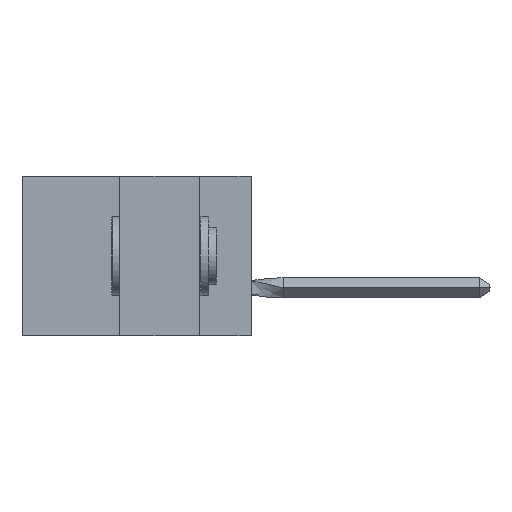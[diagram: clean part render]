
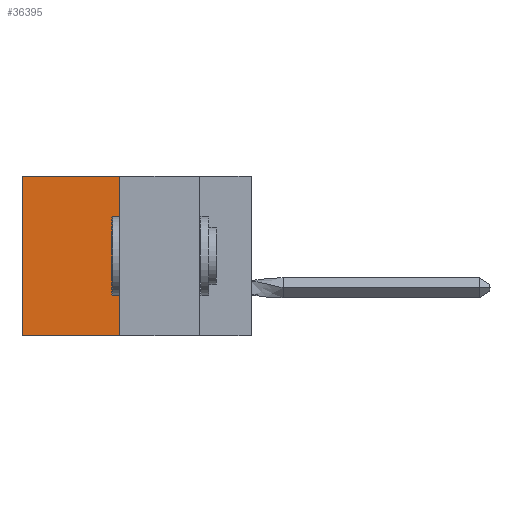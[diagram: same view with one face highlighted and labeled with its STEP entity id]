
A CAD part, left-side view. The second image highlights one B-rep face of the part: STEP entity #36395.
In plain terms, the highlighted planar face has unit normal (-1, 0, 0).
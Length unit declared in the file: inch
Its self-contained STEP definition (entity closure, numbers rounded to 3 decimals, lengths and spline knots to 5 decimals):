
#522 = ORIENTED_EDGE ( 'NONE', *, *, #19069, .T. ) ;
#924 = DIRECTION ( 'NONE',  ( 0., 0., -1. ) ) ;
#5753 = CARTESIAN_POINT ( 'NONE',  ( 0.305, 0.413, 0. ) ) ;
#6924 = AXIS2_PLACEMENT_3D ( 'NONE', #22891, #28687, #8133 ) ;
#8133 = DIRECTION ( 'NONE',  ( 0., 0., -1. ) ) ;
#8919 = DIRECTION ( 'NONE',  ( 0., 1., 0. ) ) ;
#9154 = LINE ( 'NONE', #21978, #22723 ) ;
#9664 = EDGE_CURVE ( 'NONE', #28384, #33507, #21835, .T. ) ;
#10428 = EDGE_LOOP ( 'NONE', ( #23307, #26451, #27748, #522 ) ) ;
#12015 = VECTOR ( 'NONE', #17078, 39.37008 ) ;
#12724 = VERTEX_POINT ( 'NONE', #27135 ) ;
#14431 = EDGE_CURVE ( 'NONE', #22298, #12724, #25106, .T. ) ;
#17039 = LINE ( 'NONE', #5753, #33776 ) ;
#17078 = DIRECTION ( 'NONE',  ( 0., 0., -1. ) ) ;
#19069 = EDGE_CURVE ( 'NONE', #28384, #22298, #17039, .T. ) ;
#20047 = FACE_OUTER_BOUND ( 'NONE', #10428, .T. ) ;
#21722 = EDGE_CURVE ( 'NONE', #33507, #12724, #9154, .T. ) ;
#21835 = LINE ( 'NONE', #30647, #29684 ) ;
#21978 = CARTESIAN_POINT ( 'NONE',  ( 0.305, 0.413, -0.5 ) ) ;
#22298 = VERTEX_POINT ( 'NONE', #22511 ) ;
#22511 = CARTESIAN_POINT ( 'NONE',  ( 0.305, 0.72, 0. ) ) ;
#22723 = VECTOR ( 'NONE', #24967, 39.37008 ) ;
#22752 = PLANE ( 'NONE',  #6924 ) ;
#22891 = CARTESIAN_POINT ( 'NONE',  ( 0.305, 0.413, -0.5 ) ) ;
#23307 = ORIENTED_EDGE ( 'NONE', *, *, #14431, .T. ) ;
#24967 = DIRECTION ( 'NONE',  ( 0., 1., 0. ) ) ;
#25106 = LINE ( 'NONE', #37203, #12015 ) ;
#26451 = ORIENTED_EDGE ( 'NONE', *, *, #21722, .F. ) ;
#27135 = CARTESIAN_POINT ( 'NONE',  ( 0.305, 0.72, -0.5 ) ) ;
#27748 = ORIENTED_EDGE ( 'NONE', *, *, #9664, .F. ) ;
#28384 = VERTEX_POINT ( 'NONE', #31563 ) ;
#28687 = DIRECTION ( 'NONE',  ( 1., 0., 0. ) ) ;
#29684 = VECTOR ( 'NONE', #924, 39.37008 ) ;
#30647 = CARTESIAN_POINT ( 'NONE',  ( 0.305, 0.413, -0.5 ) ) ;
#31563 = CARTESIAN_POINT ( 'NONE',  ( 0.305, 0.413, 0. ) ) ;
#33117 = CARTESIAN_POINT ( 'NONE',  ( 0.305, 0.413, -0.5 ) ) ;
#33507 = VERTEX_POINT ( 'NONE', #33117 ) ;
#33776 = VECTOR ( 'NONE', #8919, 39.37008 ) ;
#36395 = ADVANCED_FACE ( 'NONE', ( #20047 ), #22752, .F. ) ;
#37203 = CARTESIAN_POINT ( 'NONE',  ( 0.305, 0.72, -0.5 ) ) ;
